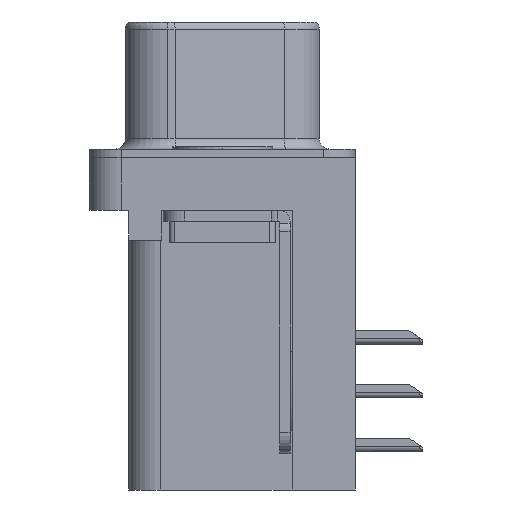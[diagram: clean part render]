
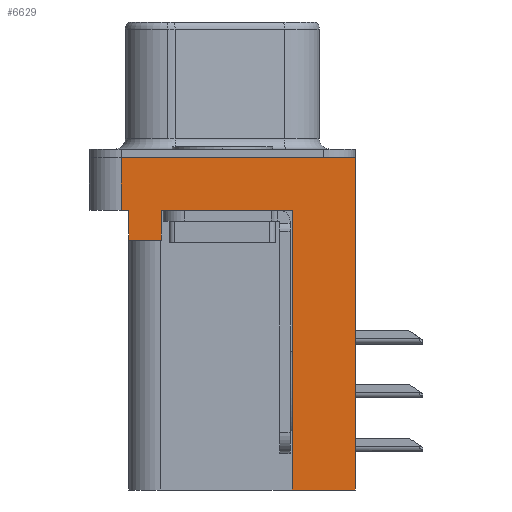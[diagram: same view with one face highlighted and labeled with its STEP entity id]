
A CAD part, left-side view. The second image highlights one B-rep face of the part: STEP entity #6629.
In plain terms, the highlighted planar face has unit normal (-1, 0, 0).
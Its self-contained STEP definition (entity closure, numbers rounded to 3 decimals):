
#168 = EDGE_CURVE ( 'NONE', #473, #18488, #13590, .T. ) ;
#473 = VERTEX_POINT ( 'NONE', #13504 ) ;
#825 = LINE ( 'NONE', #21833, #10399 ) ;
#888 = ORIENTED_EDGE ( 'NONE', *, *, #10991, .F. ) ;
#979 = DIRECTION ( 'NONE',  ( 0., 0., 1. ) ) ;
#1533 = DIRECTION ( 'NONE',  ( 0., 0., 1. ) ) ;
#1943 = EDGE_CURVE ( 'NONE', #12621, #17685, #17190, .T. ) ;
#2257 = VECTOR ( 'NONE', #21923, 1000. ) ;
#2585 = VECTOR ( 'NONE', #3776, 1000. ) ;
#3315 = ORIENTED_EDGE ( 'NONE', *, *, #13604, .T. ) ;
#3338 = LINE ( 'NONE', #4002, #17022 ) ;
#3776 = DIRECTION ( 'NONE',  ( 0., 0., 1. ) ) ;
#3920 = CARTESIAN_POINT ( 'NONE',  ( -2.935, 4.425, -3.9 ) ) ;
#4002 = CARTESIAN_POINT ( 'NONE',  ( -2.935, -6.275, 0. ) ) ;
#4043 = EDGE_CURVE ( 'NONE', #18616, #17685, #825, .T. ) ;
#4193 = VERTEX_POINT ( 'NONE', #9566 ) ;
#4649 = CARTESIAN_POINT ( 'NONE',  ( -2.935, 2.895, -3.9 ) ) ;
#4715 = PLANE ( 'NONE',  #19720 ) ;
#4810 = EDGE_CURVE ( 'NONE', #8253, #473, #14243, .T. ) ;
#5100 = CARTESIAN_POINT ( 'NONE',  ( -2.935, -3.295, -15.7 ) ) ;
#5103 = CARTESIAN_POINT ( 'NONE',  ( -2.935, -3.295, -15.7 ) ) ;
#5499 = CARTESIAN_POINT ( 'NONE',  ( -2.935, 4.425, -2.5 ) ) ;
#5765 = ORIENTED_EDGE ( 'NONE', *, *, #16758, .F. ) ;
#6616 = DIRECTION ( 'NONE',  ( 0., 0., 1. ) ) ;
#6629 = ADVANCED_FACE ( 'NONE', ( #21081 ), #4715, .T. ) ;
#6883 = LINE ( 'NONE', #10702, #20535 ) ;
#6949 = LINE ( 'NONE', #4649, #11057 ) ;
#8219 = VERTEX_POINT ( 'NONE', #17519 ) ;
#8253 = VERTEX_POINT ( 'NONE', #15824 ) ;
#8865 = VECTOR ( 'NONE', #19937, 1000. ) ;
#9323 = CARTESIAN_POINT ( 'NONE',  ( -2.935, 2.895, -2.5 ) ) ;
#9351 = DIRECTION ( 'NONE',  ( 0., 1., 0. ) ) ;
#9449 = ORIENTED_EDGE ( 'NONE', *, *, #4810, .F. ) ;
#9566 = CARTESIAN_POINT ( 'NONE',  ( -2.935, -6.275, 0. ) ) ;
#9578 = EDGE_CURVE ( 'NONE', #13636, #18488, #11705, .T. ) ;
#10399 = VECTOR ( 'NONE', #21259, 1000. ) ;
#10507 = CARTESIAN_POINT ( 'NONE',  ( -2.935, 4.775, 0. ) ) ;
#10702 = CARTESIAN_POINT ( 'NONE',  ( -2.935, -6.275, -2.5 ) ) ;
#10991 = EDGE_CURVE ( 'NONE', #8219, #12621, #17587, .T. ) ;
#11057 = VECTOR ( 'NONE', #979, 1000. ) ;
#11125 = CARTESIAN_POINT ( 'NONE',  ( -2.935, 4.425, -3.9 ) ) ;
#11151 = CARTESIAN_POINT ( 'NONE',  ( -2.935, -6.275, -2.5 ) ) ;
#11191 = VECTOR ( 'NONE', #9351, 1000. ) ;
#11348 = ORIENTED_EDGE ( 'NONE', *, *, #15789, .T. ) ;
#11705 = LINE ( 'NONE', #11151, #2257 ) ;
#11834 = CARTESIAN_POINT ( 'NONE',  ( -2.935, -6.275, -2.5 ) ) ;
#12198 = VECTOR ( 'NONE', #15775, 1000. ) ;
#12373 = VECTOR ( 'NONE', #1533, 1000. ) ;
#12621 = VERTEX_POINT ( 'NONE', #12893 ) ;
#12893 = CARTESIAN_POINT ( 'NONE',  ( -2.935, -3.295, -15.7 ) ) ;
#13504 = CARTESIAN_POINT ( 'NONE',  ( -2.935, 4.425, -3.9 ) ) ;
#13590 = LINE ( 'NONE', #3920, #8865 ) ;
#13600 = CARTESIAN_POINT ( 'NONE',  ( -2.935, 4.775, -2.5 ) ) ;
#13604 = EDGE_CURVE ( 'NONE', #8253, #18616, #6949, .T. ) ;
#13636 = VERTEX_POINT ( 'NONE', #13600 ) ;
#14243 = LINE ( 'NONE', #11125, #11191 ) ;
#14445 = CARTESIAN_POINT ( 'NONE',  ( -2.935, 4.775, -2.5 ) ) ;
#14661 = ORIENTED_EDGE ( 'NONE', *, *, #4043, .T. ) ;
#15313 = ORIENTED_EDGE ( 'NONE', *, *, #1943, .F. ) ;
#15775 = DIRECTION ( 'NONE',  ( 0., 1., 0. ) ) ;
#15789 = EDGE_CURVE ( 'NONE', #8219, #4193, #6883, .T. ) ;
#15824 = CARTESIAN_POINT ( 'NONE',  ( -2.935, 2.895, -3.9 ) ) ;
#16267 = LINE ( 'NONE', #14445, #2585 ) ;
#16485 = DIRECTION ( 'NONE',  ( 0., -1., 0. ) ) ;
#16758 = EDGE_CURVE ( 'NONE', #13636, #22943, #16267, .T. ) ;
#17022 = VECTOR ( 'NONE', #16485, 1000. ) ;
#17190 = LINE ( 'NONE', #5100, #12373 ) ;
#17293 = DIRECTION ( 'NONE',  ( -1., 0., 0. ) ) ;
#17401 = EDGE_LOOP ( 'NONE', ( #20491, #5765, #19144, #20758, #9449, #3315, #14661, #15313, #888, #11348 ) ) ;
#17519 = CARTESIAN_POINT ( 'NONE',  ( -2.935, -6.275, -15.7 ) ) ;
#17587 = LINE ( 'NONE', #5103, #12198 ) ;
#17685 = VERTEX_POINT ( 'NONE', #21084 ) ;
#17918 = DIRECTION ( 'NONE',  ( 0., 0., 1. ) ) ;
#18488 = VERTEX_POINT ( 'NONE', #5499 ) ;
#18616 = VERTEX_POINT ( 'NONE', #9323 ) ;
#19144 = ORIENTED_EDGE ( 'NONE', *, *, #9578, .T. ) ;
#19720 = AXIS2_PLACEMENT_3D ( 'NONE', #11834, #17293, #6616 ) ;
#19937 = DIRECTION ( 'NONE',  ( 0., 0., 1. ) ) ;
#20369 = EDGE_CURVE ( 'NONE', #22943, #4193, #3338, .T. ) ;
#20491 = ORIENTED_EDGE ( 'NONE', *, *, #20369, .F. ) ;
#20535 = VECTOR ( 'NONE', #17918, 1000. ) ;
#20758 = ORIENTED_EDGE ( 'NONE', *, *, #168, .F. ) ;
#21081 = FACE_OUTER_BOUND ( 'NONE', #17401, .T. ) ;
#21084 = CARTESIAN_POINT ( 'NONE',  ( -2.935, -3.295, -2.5 ) ) ;
#21259 = DIRECTION ( 'NONE',  ( 0., -1., 0. ) ) ;
#21833 = CARTESIAN_POINT ( 'NONE',  ( -2.935, -6.275, -2.5 ) ) ;
#21923 = DIRECTION ( 'NONE',  ( 0., -1., 0. ) ) ;
#22943 = VERTEX_POINT ( 'NONE', #10507 ) ;
